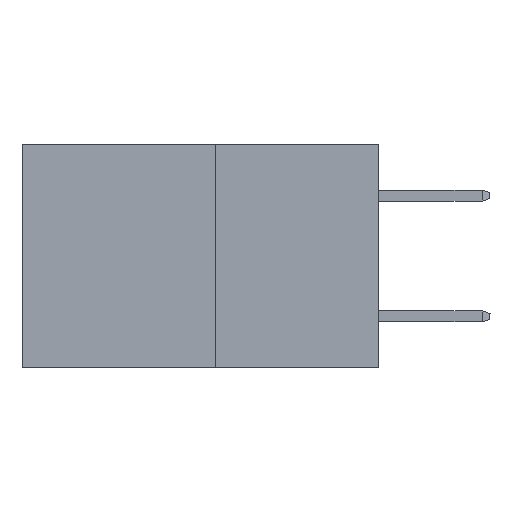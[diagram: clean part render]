
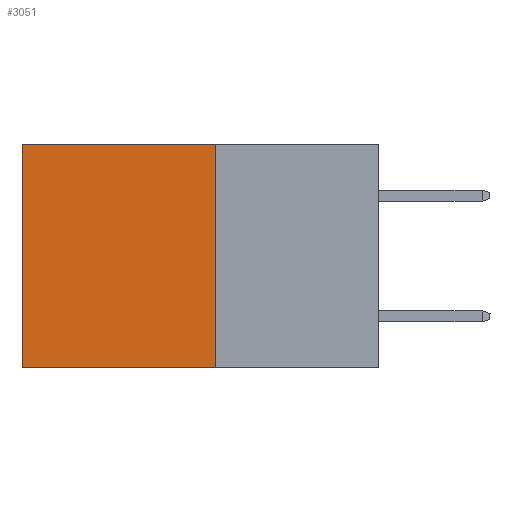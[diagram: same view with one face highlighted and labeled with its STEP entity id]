
A CAD part, left-side view. The second image highlights one B-rep face of the part: STEP entity #3051.
In plain terms, the highlighted planar face has unit normal (-1, 0, 0).
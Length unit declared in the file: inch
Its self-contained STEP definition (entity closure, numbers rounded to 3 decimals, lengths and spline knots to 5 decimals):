
#269 = AXIS2_PLACEMENT_3D ( 'NONE', #6631, #7658, #7802 ) ;
#396 = DIRECTION ( 'NONE',  ( 0., 0., -1. ) ) ;
#499 = VECTOR ( 'NONE', #9674, 39.37008 ) ;
#804 = VERTEX_POINT ( 'NONE', #3493 ) ;
#853 = ORIENTED_EDGE ( 'NONE', *, *, #1494, .F. ) ;
#1494 = EDGE_CURVE ( 'NONE', #6627, #12060, #7606, .T. ) ;
#1715 = DIRECTION ( 'NONE',  ( 0., 1., 0. ) ) ;
#1854 = CARTESIAN_POINT ( 'NONE',  ( 0.277, 0.27, 0. ) ) ;
#2273 = VECTOR ( 'NONE', #12254, 39.37008 ) ;
#2799 = ORIENTED_EDGE ( 'NONE', *, *, #3699, .T. ) ;
#3051 = ADVANCED_FACE ( 'NONE', ( #8522 ), #7706, .F. ) ;
#3493 = CARTESIAN_POINT ( 'NONE',  ( 0.277, 0.59, -0.37 ) ) ;
#3524 = CARTESIAN_POINT ( 'NONE',  ( 0.277, 0.27, -0.37 ) ) ;
#3624 = CARTESIAN_POINT ( 'NONE',  ( 0.277, 0.27, -0.37 ) ) ;
#3663 = CARTESIAN_POINT ( 'NONE',  ( 0.277, 0.59, 0. ) ) ;
#3699 = EDGE_CURVE ( 'NONE', #12096, #804, #5737, .T. ) ;
#4058 = CARTESIAN_POINT ( 'NONE',  ( 0.277, 0.59, -0.37 ) ) ;
#4091 = VECTOR ( 'NONE', #1715, 39.37008 ) ;
#4410 = LINE ( 'NONE', #4657, #4091 ) ;
#4657 = CARTESIAN_POINT ( 'NONE',  ( 0.277, 0.27, 0. ) ) ;
#5737 = LINE ( 'NONE', #4058, #499 ) ;
#6627 = VERTEX_POINT ( 'NONE', #1854 ) ;
#6631 = CARTESIAN_POINT ( 'NONE',  ( 0.277, 0.27, -0.37 ) ) ;
#7471 = LINE ( 'NONE', #8480, #2273 ) ;
#7606 = LINE ( 'NONE', #3524, #12400 ) ;
#7658 = DIRECTION ( 'NONE',  ( 1., 0., 0. ) ) ;
#7706 = PLANE ( 'NONE',  #269 ) ;
#7802 = DIRECTION ( 'NONE',  ( 0., 0., -1. ) ) ;
#7942 = ORIENTED_EDGE ( 'NONE', *, *, #10122, .T. ) ;
#8480 = CARTESIAN_POINT ( 'NONE',  ( 0.277, 0.27, -0.37 ) ) ;
#8522 = FACE_OUTER_BOUND ( 'NONE', #10476, .T. ) ;
#9417 = EDGE_CURVE ( 'NONE', #12060, #804, #7471, .T. ) ;
#9674 = DIRECTION ( 'NONE',  ( 0., 0., -1. ) ) ;
#10122 = EDGE_CURVE ( 'NONE', #6627, #12096, #4410, .T. ) ;
#10476 = EDGE_LOOP ( 'NONE', ( #2799, #10631, #853, #7942 ) ) ;
#10631 = ORIENTED_EDGE ( 'NONE', *, *, #9417, .F. ) ;
#12060 = VERTEX_POINT ( 'NONE', #3624 ) ;
#12096 = VERTEX_POINT ( 'NONE', #3663 ) ;
#12254 = DIRECTION ( 'NONE',  ( 0., 1., 0. ) ) ;
#12400 = VECTOR ( 'NONE', #396, 39.37008 ) ;
